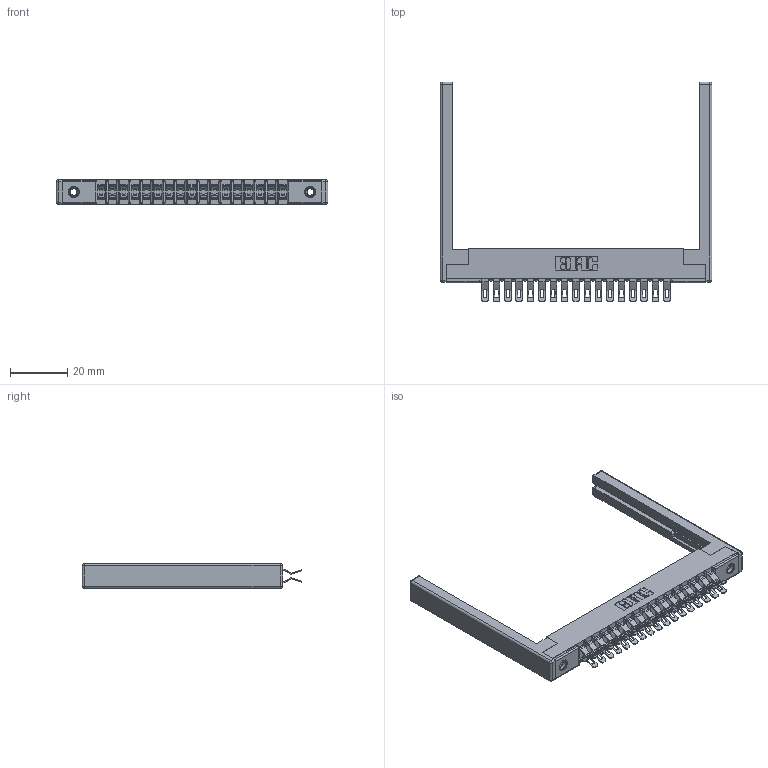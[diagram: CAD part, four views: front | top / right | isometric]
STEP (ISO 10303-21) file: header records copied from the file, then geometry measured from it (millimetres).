
FILE_DESCRIPTION (( 'STEP AP203' ), '1' );
FILE_NAME ('307-034-555-268.STEP', '2019-09-06T02:43:33', ( '' ), ( '' ), 'SwSTEP 2.0', 'SolidWorks 2016', '' );
FILE_SCHEMA (( 'CONFIG_CONTROL_DESIGN' ));
Length unit declared in the file: inch
Products named in the file (5): 307 Part_.156 Dia Mounting Holes; 307-220-068; 307-034-555-268; 307-290-001_555; 345-250-001_345-250-001-102
Assembly tree (39 placements, depth 2):
  307-034-555-268
    307 Part_.156 Dia Mounting Holes
    307-290-001_555  x34
    307-220-068  x2
    345-250-001_345-250-001-102  x2
Bounding box: 94.79 x 76.71 x 8.71 mm (x, y, z)
Volume: 10863.8 mm3; surface area: 15474.1 mm2
Topology: 39 solids, 39 shells, 2364 faces, 6867 edges, 4462 vertices
Faces by surface type: plane 1314, cylinder 990, sphere 44, cone 12, torus 4
Entity records: 21496 total; most frequent: CARTESIAN_POINT 3506, DIRECTION 3467, ORIENTED_EDGE 3466, EDGE_CURVE 1733, VECTOR 1305, LINE 1305, VERTEX_POINT 1120, AXIS2_PLACEMENT_3D 1081
